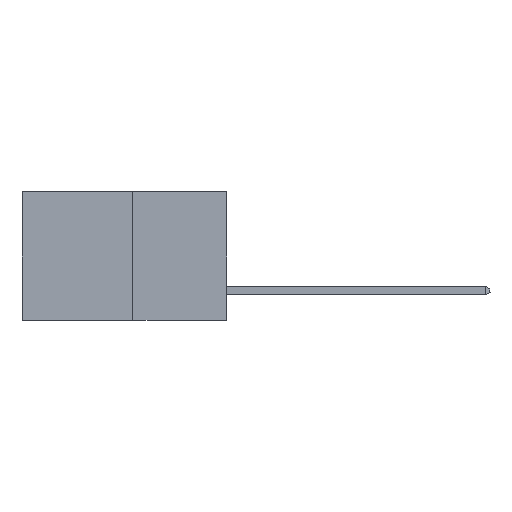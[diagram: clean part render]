
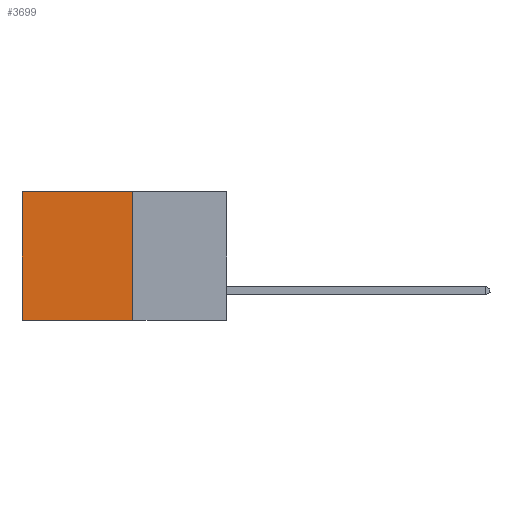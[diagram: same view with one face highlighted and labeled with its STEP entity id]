
A CAD part, left-side view. The second image highlights one B-rep face of the part: STEP entity #3699.
In plain terms, the highlighted planar face has unit normal (-1, 0, 0).
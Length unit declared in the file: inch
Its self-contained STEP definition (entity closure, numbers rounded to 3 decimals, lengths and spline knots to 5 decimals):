
#117 = VECTOR ( 'NONE', #313, 39.37008 ) ;
#313 = DIRECTION ( 'NONE',  ( 0., 1., 0. ) ) ;
#473 = AXIS2_PLACEMENT_3D ( 'NONE', #7913, #4468, #11331 ) ;
#655 = CARTESIAN_POINT ( 'NONE',  ( 0.277, 0.27, -0.37 ) ) ;
#671 = DIRECTION ( 'NONE',  ( 0., 1., 0. ) ) ;
#1366 = EDGE_CURVE ( 'NONE', #1395, #8050, #5630, .T. ) ;
#1395 = VERTEX_POINT ( 'NONE', #6500 ) ;
#1977 = VERTEX_POINT ( 'NONE', #7838 ) ;
#2816 = EDGE_CURVE ( 'NONE', #1977, #1395, #9204, .T. ) ;
#3078 = CARTESIAN_POINT ( 'NONE',  ( 0.277, 0.59, -0.37 ) ) ;
#3602 = DIRECTION ( 'NONE',  ( 0., 0., -1. ) ) ;
#3672 = CARTESIAN_POINT ( 'NONE',  ( 0.277, 0.59, -0.37 ) ) ;
#3699 = ADVANCED_FACE ( 'NONE', ( #10454 ), #10643, .F. ) ;
#4468 = DIRECTION ( 'NONE',  ( 1., 0., 0. ) ) ;
#4796 = VECTOR ( 'NONE', #3602, 39.37008 ) ;
#4899 = EDGE_CURVE ( 'NONE', #11594, #8050, #9721, .T. ) ;
#5630 = LINE ( 'NONE', #655, #10250 ) ;
#5863 = EDGE_CURVE ( 'NONE', #1977, #11594, #10266, .T. ) ;
#5866 = ORIENTED_EDGE ( 'NONE', *, *, #1366, .F. ) ;
#6172 = ORIENTED_EDGE ( 'NONE', *, *, #5863, .T. ) ;
#6500 = CARTESIAN_POINT ( 'NONE',  ( 0.277, 0.27, -0.37 ) ) ;
#7294 = CARTESIAN_POINT ( 'NONE',  ( 0.277, 0.27, -0.37 ) ) ;
#7838 = CARTESIAN_POINT ( 'NONE',  ( 0.277, 0.27, 0. ) ) ;
#7913 = CARTESIAN_POINT ( 'NONE',  ( 0.277, 0.27, -0.37 ) ) ;
#8050 = VERTEX_POINT ( 'NONE', #3078 ) ;
#8120 = EDGE_LOOP ( 'NONE', ( #10465, #5866, #8323, #6172 ) ) ;
#8323 = ORIENTED_EDGE ( 'NONE', *, *, #2816, .F. ) ;
#9204 = LINE ( 'NONE', #7294, #11572 ) ;
#9721 = LINE ( 'NONE', #3672, #4796 ) ;
#10155 = CARTESIAN_POINT ( 'NONE',  ( 0.277, 0.27, 0. ) ) ;
#10250 = VECTOR ( 'NONE', #671, 39.37008 ) ;
#10266 = LINE ( 'NONE', #10155, #117 ) ;
#10454 = FACE_OUTER_BOUND ( 'NONE', #8120, .T. ) ;
#10465 = ORIENTED_EDGE ( 'NONE', *, *, #4899, .T. ) ;
#10643 = PLANE ( 'NONE',  #473 ) ;
#11331 = DIRECTION ( 'NONE',  ( 0., 0., -1. ) ) ;
#11572 = VECTOR ( 'NONE', #11869, 39.37008 ) ;
#11594 = VERTEX_POINT ( 'NONE', #11675 ) ;
#11675 = CARTESIAN_POINT ( 'NONE',  ( 0.277, 0.59, 0. ) ) ;
#11869 = DIRECTION ( 'NONE',  ( 0., 0., -1. ) ) ;
